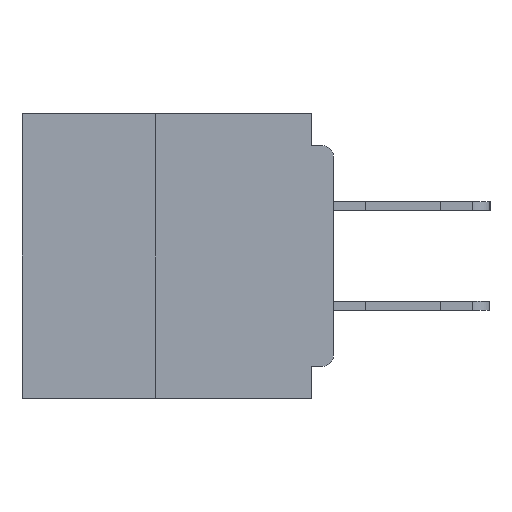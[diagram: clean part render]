
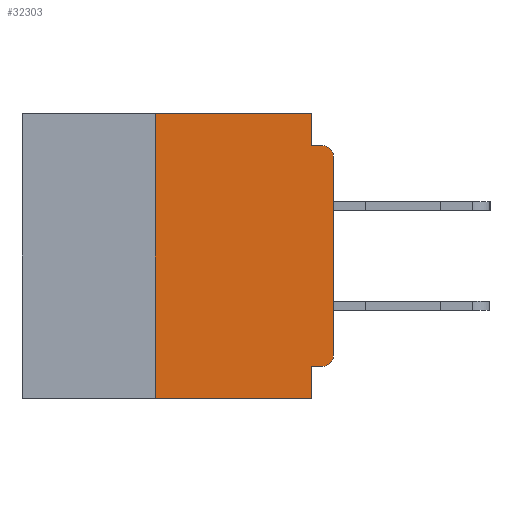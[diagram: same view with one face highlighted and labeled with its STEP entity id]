
A CAD part, left-side view. The second image highlights one B-rep face of the part: STEP entity #32303.
In plain terms, the highlighted planar face has unit normal (-1, 0, 0).
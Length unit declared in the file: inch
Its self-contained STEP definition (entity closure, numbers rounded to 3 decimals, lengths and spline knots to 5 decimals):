
#4097 = EDGE_CURVE ( 'NONE', #36568, #35212, #55756, .T. ) ;
#4794 = CARTESIAN_POINT ( 'NONE',  ( 0., 0.25, -0.4 ) ) ;
#5234 = ORIENTED_EDGE ( 'NONE', *, *, #48484, .F. ) ;
#5568 = CARTESIAN_POINT ( 'NONE',  ( 0., 0.031, -0.355 ) ) ;
#5748 = CIRCLE ( 'NONE', #23095, 0.015 ) ;
#6673 = VECTOR ( 'NONE', #52601, 39.37008 ) ;
#6754 = ORIENTED_EDGE ( 'NONE', *, *, #54756, .F. ) ;
#8766 = LINE ( 'NONE', #30967, #44055 ) ;
#9775 = CARTESIAN_POINT ( 'NONE',  ( 0., 0.015, -0.045 ) ) ;
#9934 = CARTESIAN_POINT ( 'NONE',  ( 0., 0.031, 0. ) ) ;
#11361 = ORIENTED_EDGE ( 'NONE', *, *, #41550, .T. ) ;
#11599 = DIRECTION ( 'NONE',  ( 1., 0., 0. ) ) ;
#16337 = CARTESIAN_POINT ( 'NONE',  ( 0., 0.031, -0.045 ) ) ;
#17102 = DIRECTION ( 'NONE',  ( 0., 1., 0. ) ) ;
#18459 = ORIENTED_EDGE ( 'NONE', *, *, #44950, .F. ) ;
#18813 = DIRECTION ( 'NONE',  ( 0., 0., -1. ) ) ;
#19103 = EDGE_CURVE ( 'NONE', #27307, #23400, #44540, .T. ) ;
#19531 = CARTESIAN_POINT ( 'NONE',  ( 0., 0., 0. ) ) ;
#19707 = VERTEX_POINT ( 'NONE', #33687 ) ;
#19964 = VERTEX_POINT ( 'NONE', #40264 ) ;
#20187 = EDGE_CURVE ( 'NONE', #28405, #35212, #25986, .T. ) ;
#20903 = LINE ( 'NONE', #41306, #55766 ) ;
#21323 = LINE ( 'NONE', #19531, #45582 ) ;
#21691 = VECTOR ( 'NONE', #42135, 39.37008 ) ;
#21786 = VERTEX_POINT ( 'NONE', #9775 ) ;
#22452 = DIRECTION ( 'NONE',  ( 0., -1., 0. ) ) ;
#22459 = DIRECTION ( 'NONE',  ( -1., 0., 0. ) ) ;
#22478 = DIRECTION ( 'NONE',  ( -1., 0., 0. ) ) ;
#23085 = AXIS2_PLACEMENT_3D ( 'NONE', #34591, #11599, #43744 ) ;
#23095 = AXIS2_PLACEMENT_3D ( 'NONE', #49752, #22478, #54294 ) ;
#23400 = VERTEX_POINT ( 'NONE', #16337 ) ;
#25986 = LINE ( 'NONE', #32461, #59343 ) ;
#27307 = VERTEX_POINT ( 'NONE', #51549 ) ;
#27610 = CARTESIAN_POINT ( 'NONE',  ( 0., 0.031, -0.4 ) ) ;
#27911 = ORIENTED_EDGE ( 'NONE', *, *, #4097, .T. ) ;
#28405 = VERTEX_POINT ( 'NONE', #5568 ) ;
#28745 = VECTOR ( 'NONE', #22452, 39.37008 ) ;
#29999 = PLANE ( 'NONE',  #23085 ) ;
#30020 = EDGE_CURVE ( 'NONE', #43977, #37300, #38694, .T. ) ;
#30967 = CARTESIAN_POINT ( 'NONE',  ( 0., 0., -0.355 ) ) ;
#31366 = LINE ( 'NONE', #48027, #6673 ) ;
#32303 = ADVANCED_FACE ( 'NONE', ( #38435 ), #29999, .F. ) ;
#32461 = CARTESIAN_POINT ( 'NONE',  ( 0., 0.031, -0.4 ) ) ;
#33298 = CARTESIAN_POINT ( 'NONE',  ( 0., 0., -0.34 ) ) ;
#33687 = CARTESIAN_POINT ( 'NONE',  ( 0., 0.25, 0. ) ) ;
#34591 = CARTESIAN_POINT ( 'NONE',  ( 0., 0.437, 0. ) ) ;
#35212 = VERTEX_POINT ( 'NONE', #27610 ) ;
#35383 = CARTESIAN_POINT ( 'NONE',  ( 0., 0.015, -0.355 ) ) ;
#35936 = ORIENTED_EDGE ( 'NONE', *, *, #46945, .T. ) ;
#36197 = EDGE_LOOP ( 'NONE', ( #35936, #11361, #6754, #57938, #45737, #18459, #27911, #40562, #5234, #46175 ) ) ;
#36346 = CARTESIAN_POINT ( 'NONE',  ( 0., 0.25, -0.4 ) ) ;
#36568 = VERTEX_POINT ( 'NONE', #4794 ) ;
#37300 = VERTEX_POINT ( 'NONE', #33298 ) ;
#38435 = FACE_OUTER_BOUND ( 'NONE', #36197, .T. ) ;
#38694 = CIRCLE ( 'NONE', #56524, 0.015 ) ;
#40264 = CARTESIAN_POINT ( 'NONE',  ( 0., 0., -0.06 ) ) ;
#40562 = ORIENTED_EDGE ( 'NONE', *, *, #20187, .F. ) ;
#41306 = CARTESIAN_POINT ( 'NONE',  ( 0., 0., -0.045 ) ) ;
#41550 = EDGE_CURVE ( 'NONE', #19964, #21786, #5748, .T. ) ;
#42135 = DIRECTION ( 'NONE',  ( 0., 0., -1. ) ) ;
#43744 = DIRECTION ( 'NONE',  ( 0., 0., -1. ) ) ;
#43977 = VERTEX_POINT ( 'NONE', #35383 ) ;
#44055 = VECTOR ( 'NONE', #17102, 39.37008 ) ;
#44540 = LINE ( 'NONE', #9934, #21691 ) ;
#44950 = EDGE_CURVE ( 'NONE', #36568, #19707, #47700, .T. ) ;
#45582 = VECTOR ( 'NONE', #51428, 39.37008 ) ;
#45737 = ORIENTED_EDGE ( 'NONE', *, *, #57569, .F. ) ;
#45849 = DIRECTION ( 'NONE',  ( 0., -1., 0. ) ) ;
#46175 = ORIENTED_EDGE ( 'NONE', *, *, #30020, .T. ) ;
#46945 = EDGE_CURVE ( 'NONE', #37300, #19964, #21323, .T. ) ;
#47700 = LINE ( 'NONE', #36346, #58324 ) ;
#48027 = CARTESIAN_POINT ( 'NONE',  ( 0., 0.437, 0. ) ) ;
#48484 = EDGE_CURVE ( 'NONE', #43977, #28405, #8766, .T. ) ;
#49731 = CARTESIAN_POINT ( 'NONE',  ( 0., 0.437, -0.4 ) ) ;
#49737 = CARTESIAN_POINT ( 'NONE',  ( 0., 0.015, -0.34 ) ) ;
#49752 = CARTESIAN_POINT ( 'NONE',  ( 0., 0.015, -0.06 ) ) ;
#50020 = DIRECTION ( 'NONE',  ( 0., 0., 1. ) ) ;
#51428 = DIRECTION ( 'NONE',  ( 0., 0., 1. ) ) ;
#51549 = CARTESIAN_POINT ( 'NONE',  ( 0., 0.031, 0. ) ) ;
#52601 = DIRECTION ( 'NONE',  ( 0., -1., 0. ) ) ;
#54275 = DIRECTION ( 'NONE',  ( 0., 0., -1. ) ) ;
#54294 = DIRECTION ( 'NONE',  ( 0., 0., -1. ) ) ;
#54756 = EDGE_CURVE ( 'NONE', #23400, #21786, #20903, .T. ) ;
#55756 = LINE ( 'NONE', #49731, #28745 ) ;
#55766 = VECTOR ( 'NONE', #45849, 39.37008 ) ;
#56524 = AXIS2_PLACEMENT_3D ( 'NONE', #49737, #22459, #54275 ) ;
#57569 = EDGE_CURVE ( 'NONE', #19707, #27307, #31366, .T. ) ;
#57938 = ORIENTED_EDGE ( 'NONE', *, *, #19103, .F. ) ;
#58324 = VECTOR ( 'NONE', #50020, 39.37008 ) ;
#59343 = VECTOR ( 'NONE', #18813, 39.37008 ) ;
